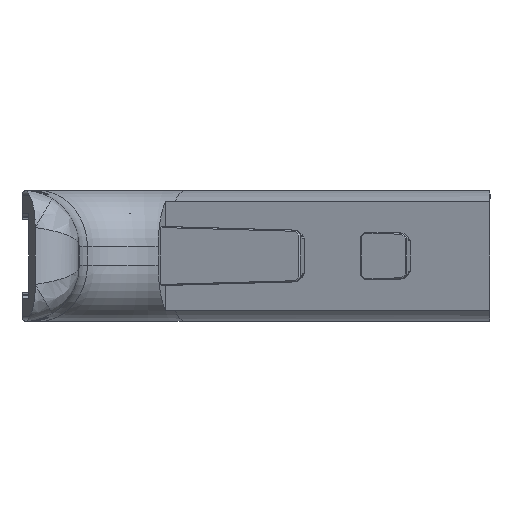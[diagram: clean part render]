
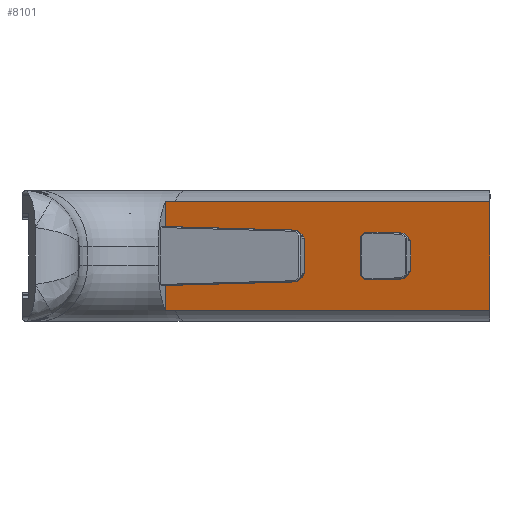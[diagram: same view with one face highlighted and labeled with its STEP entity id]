
A CAD part, left-side view. The second image highlights one B-rep face of the part: STEP entity #8101.
In plain terms, the highlighted planar face has unit normal (-0.951, 0.309, 0).
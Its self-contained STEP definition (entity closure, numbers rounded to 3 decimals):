
#478=FACE_BOUND('',#1081,.T.);
#491=B_SPLINE_CURVE_WITH_KNOTS('',3,(#11833,#11834,#11835,#11836,#11837,
#11838,#11839),.UNSPECIFIED.,.F.,.F.,(4,3,4),(0.,0.118,0.215),
 .UNSPECIFIED.);
#492=B_SPLINE_CURVE_WITH_KNOTS('',3,(#11847,#11848,#11849,#11850,#11851,
#11852,#11853),.UNSPECIFIED.,.F.,.F.,(4,3,4),(-0.215,-0.118,
0.),.UNSPECIFIED.);
#634=FACE_OUTER_BOUND('',#1080,.T.);
#1080=EDGE_LOOP('',(#5536,#5537,#5538,#5539,#5540,#5541,#5542,#5543,#5544,
#5545,#5546,#5547));
#1081=EDGE_LOOP('',(#5548,#5549,#5550,#5551,#5552,#5553,#5554,#5555,#5556));
#1574=LINE('',#11722,#2451);
#1592=LINE('',#11760,#2469);
#1600=LINE('',#11777,#2477);
#1605=LINE('',#11786,#2482);
#1607=LINE('',#11789,#2484);
#1609=LINE('',#11794,#2486);
#1611=LINE('',#11798,#2488);
#1613=LINE('',#11801,#2490);
#1615=LINE('',#11805,#2492);
#1616=LINE('',#11807,#2493);
#1622=LINE('',#11820,#2499);
#1624=LINE('',#11824,#2501);
#1625=LINE('',#11827,#2502);
#1627=LINE('',#11831,#2504);
#1628=LINE('',#11841,#2505);
#1629=LINE('',#11843,#2506);
#1630=LINE('',#11845,#2507);
#1631=LINE('',#11855,#2508);
#1632=LINE('',#11856,#2509);
#2451=VECTOR('',#9401,10.);
#2469=VECTOR('',#9437,10.);
#2477=VECTOR('',#9451,10.);
#2482=VECTOR('',#9460,10.);
#2484=VECTOR('',#9464,10.);
#2486=VECTOR('',#9468,10.);
#2488=VECTOR('',#9472,10.);
#2490=VECTOR('',#9476,10.);
#2492=VECTOR('',#9480,10.);
#2493=VECTOR('',#9483,10.);
#2499=VECTOR('',#9499,10.);
#2501=VECTOR('',#9503,10.);
#2502=VECTOR('',#9506,10.);
#2504=VECTOR('',#9510,10.);
#2505=VECTOR('',#9511,10.);
#2506=VECTOR('',#9512,10.);
#2507=VECTOR('',#9513,10.);
#2508=VECTOR('',#9514,10.);
#2509=VECTOR('',#9515,10.);
#3297=VERTEX_POINT('',#11719);
#3298=VERTEX_POINT('',#11721);
#3308=VERTEX_POINT('',#11757);
#3309=VERTEX_POINT('',#11759);
#3314=VERTEX_POINT('',#11774);
#3315=VERTEX_POINT('',#11776);
#3317=VERTEX_POINT('',#11785);
#3318=VERTEX_POINT('',#11791);
#3319=VERTEX_POINT('',#11793);
#3320=VERTEX_POINT('',#11797);
#3321=VERTEX_POINT('',#11803);
#3323=VERTEX_POINT('',#11818);
#3324=VERTEX_POINT('',#11822);
#3325=VERTEX_POINT('',#11826);
#3326=VERTEX_POINT('',#11830);
#3327=VERTEX_POINT('',#11832);
#3328=VERTEX_POINT('',#11840);
#3329=VERTEX_POINT('',#11842);
#3330=VERTEX_POINT('',#11844);
#3331=VERTEX_POINT('',#11846);
#3332=VERTEX_POINT('',#11854);
#4120=EDGE_CURVE('',#3298,#3297,#1574,.T.);
#4138=EDGE_CURVE('',#3308,#3309,#1592,.T.);
#4146=EDGE_CURVE('',#3314,#3315,#1600,.F.);
#4151=EDGE_CURVE('',#3298,#3317,#1605,.F.);
#4153=EDGE_CURVE('',#3314,#3317,#1607,.T.);
#4155=EDGE_CURVE('',#3318,#3319,#1609,.F.);
#4157=EDGE_CURVE('',#3320,#3319,#1611,.T.);
#4159=EDGE_CURVE('',#3318,#3315,#1613,.T.);
#4161=EDGE_CURVE('',#3321,#3297,#1615,.F.);
#4162=EDGE_CURVE('',#3320,#3321,#1616,.F.);
#4168=EDGE_CURVE('',#3323,#3308,#1622,.F.);
#4170=EDGE_CURVE('',#3323,#3324,#1624,.T.);
#4171=EDGE_CURVE('',#3309,#3325,#1625,.F.);
#4173=EDGE_CURVE('',#3326,#3324,#1627,.T.);
#4174=EDGE_CURVE('',#3327,#3326,#491,.T.);
#4175=EDGE_CURVE('',#3328,#3327,#1628,.T.);
#4176=EDGE_CURVE('',#3329,#3328,#1629,.T.);
#4177=EDGE_CURVE('',#3330,#3329,#1630,.T.);
#4178=EDGE_CURVE('',#3331,#3330,#492,.T.);
#4179=EDGE_CURVE('',#3332,#3331,#1631,.T.);
#4180=EDGE_CURVE('',#3332,#3325,#1632,.T.);
#5536=ORIENTED_EDGE('',*,*,#4170,.T.);
#5537=ORIENTED_EDGE('',*,*,#4173,.F.);
#5538=ORIENTED_EDGE('',*,*,#4174,.F.);
#5539=ORIENTED_EDGE('',*,*,#4175,.F.);
#5540=ORIENTED_EDGE('',*,*,#4176,.F.);
#5541=ORIENTED_EDGE('',*,*,#4177,.F.);
#5542=ORIENTED_EDGE('',*,*,#4178,.F.);
#5543=ORIENTED_EDGE('',*,*,#4179,.F.);
#5544=ORIENTED_EDGE('',*,*,#4180,.T.);
#5545=ORIENTED_EDGE('',*,*,#4171,.F.);
#5546=ORIENTED_EDGE('',*,*,#4138,.F.);
#5547=ORIENTED_EDGE('',*,*,#4168,.F.);
#5548=ORIENTED_EDGE('',*,*,#4120,.T.);
#5549=ORIENTED_EDGE('',*,*,#4161,.F.);
#5550=ORIENTED_EDGE('',*,*,#4162,.F.);
#5551=ORIENTED_EDGE('',*,*,#4157,.T.);
#5552=ORIENTED_EDGE('',*,*,#4155,.F.);
#5553=ORIENTED_EDGE('',*,*,#4159,.T.);
#5554=ORIENTED_EDGE('',*,*,#4146,.F.);
#5555=ORIENTED_EDGE('',*,*,#4153,.T.);
#5556=ORIENTED_EDGE('',*,*,#4151,.F.);
#7820=PLANE('',#8596);
#8101=ADVANCED_FACE('',(#634,#478),#7820,.T.);
#8596=AXIS2_PLACEMENT_3D('',#11829,#9508,#9509);
#9401=DIRECTION('',(0.,0.,1.));
#9437=DIRECTION('',(0.,0.,1.));
#9451=DIRECTION('',(0.216,0.664,-0.716));
#9460=DIRECTION('',(0.221,0.681,0.698));
#9464=DIRECTION('',(0.309,0.951,-0.026));
#9468=DIRECTION('',(-0.216,-0.664,-0.716));
#9472=DIRECTION('',(-0.309,-0.951,-0.026));
#9476=DIRECTION('',(0.,0.,-1.));
#9480=DIRECTION('',(-0.12,-0.37,0.921));
#9483=DIRECTION('',(-0.221,-0.681,0.698));
#9499=DIRECTION('',(0.216,0.664,-0.716));
#9503=DIRECTION('',(0.309,0.951,-0.026));
#9506=DIRECTION('',(-0.216,-0.664,-0.716));
#9508=DIRECTION('center_axis',(-0.951,0.309,0.));
#9509=DIRECTION('ref_axis',(0.,0.,
1.));
#9510=DIRECTION('',(0.,0.,1.));
#9511=DIRECTION('',(0.309,0.951,0.));
#9512=DIRECTION('',(0.,0.,-1.));
#9513=DIRECTION('',(-0.309,-0.951,0.));
#9514=DIRECTION('',(0.,0.,1.));
#9515=DIRECTION('',(-0.309,-0.951,-0.026));
#11719=CARTESIAN_POINT('',(-73.564,-22.449,-16.134));
#11721=CARTESIAN_POINT('',(-73.564,-22.449,-23.116));
#11722=CARTESIAN_POINT('',(-73.564,-22.449,-19.5));
#11757=CARTESIAN_POINT('',(-69.247,-9.163,-23.482));
#11759=CARTESIAN_POINT('',(-69.247,-9.163,-15.518));
#11760=CARTESIAN_POINT('',(-69.247,-9.163,-23.25));
#11774=CARTESIAN_POINT('',(-76.827,-32.493,-23.09));
#11776=CARTESIAN_POINT('',(-76.904,-32.73,-22.833));
#11777=CARTESIAN_POINT('',(-75.966,-29.843,-25.95));
#11785=CARTESIAN_POINT('',(-73.641,-22.687,-23.36));
#11786=CARTESIAN_POINT('',(-72.921,-20.471,-21.09));
#11789=CARTESIAN_POINT('',(-77.392,-34.23,-23.042));
#11791=CARTESIAN_POINT('',(-76.904,-32.73,-16.167));
#11793=CARTESIAN_POINT('',(-76.827,-32.493,-15.91));
#11794=CARTESIAN_POINT('',(-75.966,-29.843,-13.05));
#11797=CARTESIAN_POINT('',(-73.641,-22.687,-15.64));
#11798=CARTESIAN_POINT('',(-77.392,-34.23,-15.958));
#11801=CARTESIAN_POINT('',(-76.904,-32.73,-22.834));
#11803=CARTESIAN_POINT('',(-73.619,-22.619,-15.709));
#11805=CARTESIAN_POINT('',(-73.279,-21.571,-18.321));
#11807=CARTESIAN_POINT('',(-72.921,-20.471,-17.91));
#11818=CARTESIAN_POINT('',(-69.169,-8.925,-23.738));
#11820=CARTESIAN_POINT('',(-70.223,-12.167,-20.239));
#11822=CARTESIAN_POINT('',(-59.244,21.623,-24.579));
#11824=CARTESIAN_POINT('',(-77.392,-34.23,-23.042));
#11826=CARTESIAN_POINT('',(-69.169,-8.925,-15.262));
#11827=CARTESIAN_POINT('',(-70.223,-12.167,-18.761));
#11829=CARTESIAN_POINT('Origin',(-72.072,-17.859,-19.5));
#11830=CARTESIAN_POINT('',(-59.244,21.623,-31.647));
#11831=CARTESIAN_POINT('',(-59.244,21.623,-26.168));
#11832=CARTESIAN_POINT('',(-59.924,19.53,-31.56));
#11833=CARTESIAN_POINT('Ctrl Pts',(-59.924,19.53,-31.56));
#11834=CARTESIAN_POINT('Ctrl Pts',(-59.802,19.905,-31.56));
#11835=CARTESIAN_POINT('Ctrl Pts',(-59.678,20.286,-31.568));
#11836=CARTESIAN_POINT('Ctrl Pts',(-59.553,20.671,-31.586));
#11837=CARTESIAN_POINT('Ctrl Pts',(-59.45,20.99,-31.6));
#11838=CARTESIAN_POINT('Ctrl Pts',(-59.347,21.306,-31.621));
#11839=CARTESIAN_POINT('Ctrl Pts',(-59.244,21.623,-31.647));
#11840=CARTESIAN_POINT('',(-82.59,-50.229,-31.56));
#11841=CARTESIAN_POINT('',(-55.801,32.217,-31.56));
#11842=CARTESIAN_POINT('',(-82.59,-50.229,-7.44));
#11843=CARTESIAN_POINT('',(-82.59,-50.229,-9.75));
#11844=CARTESIAN_POINT('',(-59.924,19.53,-7.44));
#11845=CARTESIAN_POINT('',(-68.34,-6.372,-7.44));
#11846=CARTESIAN_POINT('',(-59.244,21.623,-7.353));
#11847=CARTESIAN_POINT('Ctrl Pts',(-59.244,21.623,-7.353));
#11848=CARTESIAN_POINT('Ctrl Pts',(-59.347,21.306,-7.379));
#11849=CARTESIAN_POINT('Ctrl Pts',(-59.45,20.99,-7.4));
#11850=CARTESIAN_POINT('Ctrl Pts',(-59.553,20.671,-7.414));
#11851=CARTESIAN_POINT('Ctrl Pts',(-59.678,20.286,-7.432));
#11852=CARTESIAN_POINT('Ctrl Pts',(-59.802,19.905,-7.44));
#11853=CARTESIAN_POINT('Ctrl Pts',(-59.924,19.53,-7.44));
#11854=CARTESIAN_POINT('',(-59.244,21.623,-14.421));
#11855=CARTESIAN_POINT('',(-59.244,21.623,-19.5));
#11856=CARTESIAN_POINT('',(-77.392,-34.23,-15.958));
